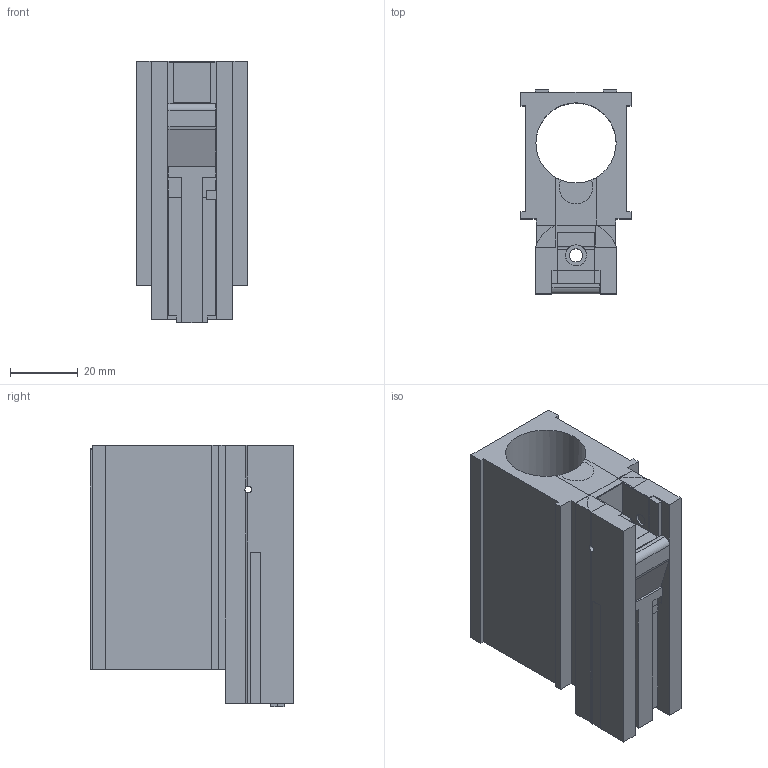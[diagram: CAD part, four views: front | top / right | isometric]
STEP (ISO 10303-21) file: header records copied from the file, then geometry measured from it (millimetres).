
FILE_DESCRIPTION(('FreeCAD Model'),'2;1');
FILE_NAME('bolt housing.step', '2015-07-10T13:10:28',('Author'),(''), 'Open CASCADE STEP processor 6.8','FreeCAD','Unknown');
FILE_SCHEMA(('AUTOMOTIVE_DESIGN_CC2 { 1 2 10303 214 -1 1 5 4 }'));
Length unit declared in the file: millimetre
Products named in the file (1): Pad016
Bounding box: 32.5 x 60.21 x 77.2 mm (x, y, z)
Volume: 66635.8 mm3; surface area: 24844.2 mm2
Topology: 1 solids, 1 shells, 195 faces, 582 edges, 387 vertices
Faces by surface type: plane 174, cylinder 17, extrusion 4
Full cylindrical faces by diameter (mm): 2 x2, 3.566 x1, 3.861 x1, 4.004 x1, 6.25 x1, 23.7 x1
Entity records: 17755 total; most frequent: CARTESIAN_POINT 7243, DIRECTION 1654, ORIENTED_EDGE 1148, PCURVE 1148, DEFINITIONAL_REPRESENTATION 1148, VECTOR 1097, LINE 1093, EDGE_CURVE 574
